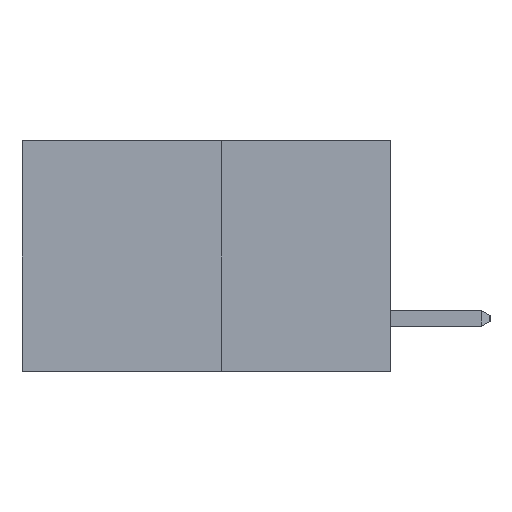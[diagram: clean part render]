
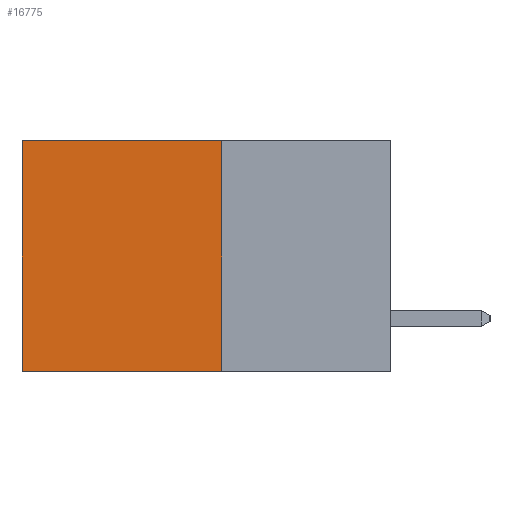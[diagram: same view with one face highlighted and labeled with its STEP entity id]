
A CAD part, left-side view. The second image highlights one B-rep face of the part: STEP entity #16775.
In plain terms, the highlighted planar face has unit normal (-1, 0, 0).
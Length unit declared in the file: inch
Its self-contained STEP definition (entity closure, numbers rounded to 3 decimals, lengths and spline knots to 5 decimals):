
#554 = VECTOR ( 'NONE', #13943, 39.37008 ) ;
#655 = EDGE_CURVE ( 'NONE', #13307, #19413, #10243, .T. ) ;
#747 = DIRECTION ( 'NONE',  ( 0., 0., -1. ) ) ;
#2036 = EDGE_LOOP ( 'NONE', ( #20487, #6822, #20085, #4110 ) ) ;
#2883 = CARTESIAN_POINT ( 'NONE',  ( 0.277, 0.59, -0.37 ) ) ;
#3208 = VECTOR ( 'NONE', #14761, 39.37008 ) ;
#4110 = ORIENTED_EDGE ( 'NONE', *, *, #18859, .T. ) ;
#6822 = ORIENTED_EDGE ( 'NONE', *, *, #655, .F. ) ;
#6925 = PLANE ( 'NONE',  #8298 ) ;
#8298 = AXIS2_PLACEMENT_3D ( 'NONE', #13659, #8669, #20293 ) ;
#8459 = LINE ( 'NONE', #2883, #9016 ) ;
#8669 = DIRECTION ( 'NONE',  ( 1., 0., 0. ) ) ;
#9016 = VECTOR ( 'NONE', #21280, 39.37008 ) ;
#10243 = LINE ( 'NONE', #19081, #554 ) ;
#10483 = CARTESIAN_POINT ( 'NONE',  ( 0.277, 0.59, 0. ) ) ;
#11841 = CARTESIAN_POINT ( 'NONE',  ( 0.277, 0.27, 0. ) ) ;
#12842 = LINE ( 'NONE', #21272, #3208 ) ;
#13307 = VERTEX_POINT ( 'NONE', #21382 ) ;
#13659 = CARTESIAN_POINT ( 'NONE',  ( 0.277, 0.27, -0.37 ) ) ;
#13943 = DIRECTION ( 'NONE',  ( 0., 1., 0. ) ) ;
#14228 = VERTEX_POINT ( 'NONE', #10483 ) ;
#14355 = CARTESIAN_POINT ( 'NONE',  ( 0.277, 0.27, -0.37 ) ) ;
#14761 = DIRECTION ( 'NONE',  ( 0., 1., 0. ) ) ;
#15334 = VERTEX_POINT ( 'NONE', #11841 ) ;
#15697 = EDGE_CURVE ( 'NONE', #15334, #13307, #17864, .T. ) ;
#16012 = FACE_OUTER_BOUND ( 'NONE', #2036, .T. ) ;
#16775 = ADVANCED_FACE ( 'NONE', ( #16012 ), #6925, .F. ) ;
#16825 = VECTOR ( 'NONE', #747, 39.37008 ) ;
#17864 = LINE ( 'NONE', #14355, #16825 ) ;
#18859 = EDGE_CURVE ( 'NONE', #15334, #14228, #12842, .T. ) ;
#19081 = CARTESIAN_POINT ( 'NONE',  ( 0.277, 0.27, -0.37 ) ) ;
#19413 = VERTEX_POINT ( 'NONE', #19433 ) ;
#19433 = CARTESIAN_POINT ( 'NONE',  ( 0.277, 0.59, -0.37 ) ) ;
#20085 = ORIENTED_EDGE ( 'NONE', *, *, #15697, .F. ) ;
#20293 = DIRECTION ( 'NONE',  ( 0., 0., -1. ) ) ;
#20487 = ORIENTED_EDGE ( 'NONE', *, *, #21636, .T. ) ;
#21272 = CARTESIAN_POINT ( 'NONE',  ( 0.277, 0.27, 0. ) ) ;
#21280 = DIRECTION ( 'NONE',  ( 0., 0., -1. ) ) ;
#21382 = CARTESIAN_POINT ( 'NONE',  ( 0.277, 0.27, -0.37 ) ) ;
#21636 = EDGE_CURVE ( 'NONE', #14228, #19413, #8459, .T. ) ;
